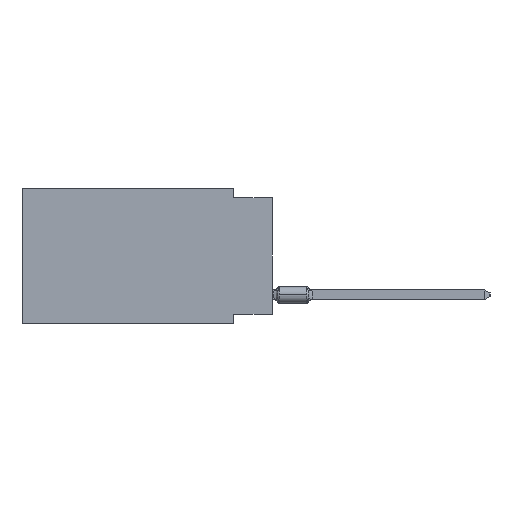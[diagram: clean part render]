
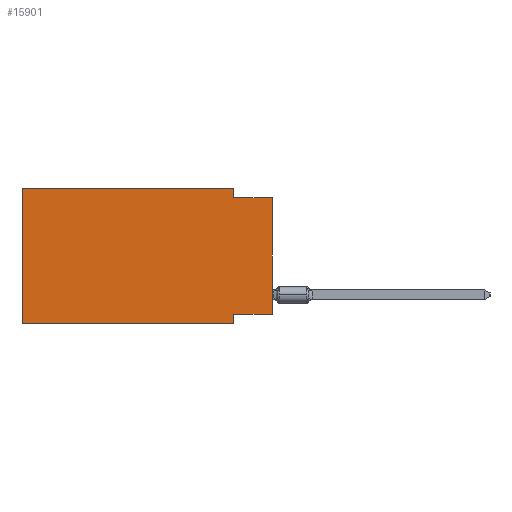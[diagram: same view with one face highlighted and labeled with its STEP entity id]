
A CAD part, left-side view. The second image highlights one B-rep face of the part: STEP entity #15901.
In plain terms, the highlighted planar face has unit normal (-1, 0, 0).
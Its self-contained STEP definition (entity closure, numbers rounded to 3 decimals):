
#1024 = CARTESIAN_POINT ( 'NONE',  ( 0., 0., -8.255 ) ) ;
#1100 = ORIENTED_EDGE ( 'NONE', *, *, #20105, .F. ) ;
#1291 = CARTESIAN_POINT ( 'NONE',  ( 0., 16.383, 0. ) ) ;
#1421 = CARTESIAN_POINT ( 'NONE',  ( 0., 0., 0. ) ) ;
#1658 = VECTOR ( 'NONE', #36488, 1000. ) ;
#1906 = VECTOR ( 'NONE', #36005, 1000. ) ;
#1938 = PLANE ( 'NONE',  #18169 ) ;
#2394 = CARTESIAN_POINT ( 'NONE',  ( 0., 16.383, -8.89 ) ) ;
#2785 = VERTEX_POINT ( 'NONE', #7102 ) ;
#5718 = VERTEX_POINT ( 'NONE', #15290 ) ;
#6500 = EDGE_CURVE ( 'NONE', #21078, #13584, #25174, .T. ) ;
#7102 = CARTESIAN_POINT ( 'NONE',  ( 0., 2.54, -8.89 ) ) ;
#8869 = EDGE_CURVE ( 'NONE', #15788, #13584, #18661, .T. ) ;
#9267 = DIRECTION ( 'NONE',  ( 0., -1., 0. ) ) ;
#9405 = CARTESIAN_POINT ( 'NONE',  ( 0., 2.54, 0. ) ) ;
#9665 = DIRECTION ( 'NONE',  ( 0., -1., 0. ) ) ;
#9977 = DIRECTION ( 'NONE',  ( 0., 0., 1. ) ) ;
#10204 = DIRECTION ( 'NONE',  ( 0., 0., 1. ) ) ;
#10760 = LINE ( 'NONE', #13714, #18590 ) ;
#11089 = VECTOR ( 'NONE', #9665, 1000. ) ;
#11866 = LINE ( 'NONE', #23166, #36573 ) ;
#12428 = VERTEX_POINT ( 'NONE', #19695 ) ;
#12626 = LINE ( 'NONE', #18360, #11089 ) ;
#13381 = LINE ( 'NONE', #24696, #1906 ) ;
#13584 = VERTEX_POINT ( 'NONE', #22632 ) ;
#13714 = CARTESIAN_POINT ( 'NONE',  ( 0., 0., -8.255 ) ) ;
#13861 = EDGE_CURVE ( 'NONE', #21308, #5718, #35400, .T. ) ;
#14257 = EDGE_LOOP ( 'NONE', ( #34477, #25440, #17973, #21934, #32396, #23883, #1100, #25215 ) ) ;
#15290 = CARTESIAN_POINT ( 'NONE',  ( 0., 16.383, 0. ) ) ;
#15788 = VERTEX_POINT ( 'NONE', #1024 ) ;
#15901 = ADVANCED_FACE ( 'NONE', ( #24922 ), #1938, .F. ) ;
#16633 = EDGE_CURVE ( 'NONE', #5718, #12428, #12626, .T. ) ;
#17034 = VECTOR ( 'NONE', #10204, 1000. ) ;
#17973 = ORIENTED_EDGE ( 'NONE', *, *, #29793, .F. ) ;
#18169 = AXIS2_PLACEMENT_3D ( 'NONE', #36231, #33434, #19347 ) ;
#18360 = CARTESIAN_POINT ( 'NONE',  ( 0., 16.383, 0. ) ) ;
#18590 = VECTOR ( 'NONE', #22058, 1000. ) ;
#18661 = LINE ( 'NONE', #1421, #32532 ) ;
#18750 = CARTESIAN_POINT ( 'NONE',  ( 0., 2.54, -0.635 ) ) ;
#19347 = DIRECTION ( 'NONE',  ( 0., 0., -1. ) ) ;
#19695 = CARTESIAN_POINT ( 'NONE',  ( 0., 2.54, 0. ) ) ;
#20105 = EDGE_CURVE ( 'NONE', #29529, #2785, #13381, .T. ) ;
#21078 = VERTEX_POINT ( 'NONE', #18750 ) ;
#21308 = VERTEX_POINT ( 'NONE', #2394 ) ;
#21934 = ORIENTED_EDGE ( 'NONE', *, *, #16633, .F. ) ;
#22058 = DIRECTION ( 'NONE',  ( 0., 1., 0. ) ) ;
#22632 = CARTESIAN_POINT ( 'NONE',  ( 0., 0., -0.635 ) ) ;
#23166 = CARTESIAN_POINT ( 'NONE',  ( 0., 16.383, -8.89 ) ) ;
#23883 = ORIENTED_EDGE ( 'NONE', *, *, #30759, .T. ) ;
#24192 = EDGE_CURVE ( 'NONE', #15788, #29529, #10760, .T. ) ;
#24265 = CARTESIAN_POINT ( 'NONE',  ( 0., 2.54, -8.255 ) ) ;
#24696 = CARTESIAN_POINT ( 'NONE',  ( 0., 2.54, -8.89 ) ) ;
#24922 = FACE_OUTER_BOUND ( 'NONE', #14257, .T. ) ;
#25174 = LINE ( 'NONE', #33166, #1658 ) ;
#25215 = ORIENTED_EDGE ( 'NONE', *, *, #24192, .F. ) ;
#25440 = ORIENTED_EDGE ( 'NONE', *, *, #6500, .F. ) ;
#29043 = DIRECTION ( 'NONE',  ( 0., 0., -1. ) ) ;
#29529 = VERTEX_POINT ( 'NONE', #24265 ) ;
#29793 = EDGE_CURVE ( 'NONE', #12428, #21078, #34240, .T. ) ;
#30759 = EDGE_CURVE ( 'NONE', #21308, #2785, #11866, .T. ) ;
#32396 = ORIENTED_EDGE ( 'NONE', *, *, #13861, .F. ) ;
#32532 = VECTOR ( 'NONE', #9977, 1000. ) ;
#33166 = CARTESIAN_POINT ( 'NONE',  ( 0., 0., -0.635 ) ) ;
#33434 = DIRECTION ( 'NONE',  ( 1., 0., 0. ) ) ;
#34240 = LINE ( 'NONE', #9405, #35339 ) ;
#34477 = ORIENTED_EDGE ( 'NONE', *, *, #8869, .T. ) ;
#35339 = VECTOR ( 'NONE', #29043, 1000. ) ;
#35400 = LINE ( 'NONE', #1291, #17034 ) ;
#36005 = DIRECTION ( 'NONE',  ( 0., 0., -1. ) ) ;
#36231 = CARTESIAN_POINT ( 'NONE',  ( 0., 16.383, 0. ) ) ;
#36488 = DIRECTION ( 'NONE',  ( 0., -1., 0. ) ) ;
#36573 = VECTOR ( 'NONE', #9267, 1000. ) ;
